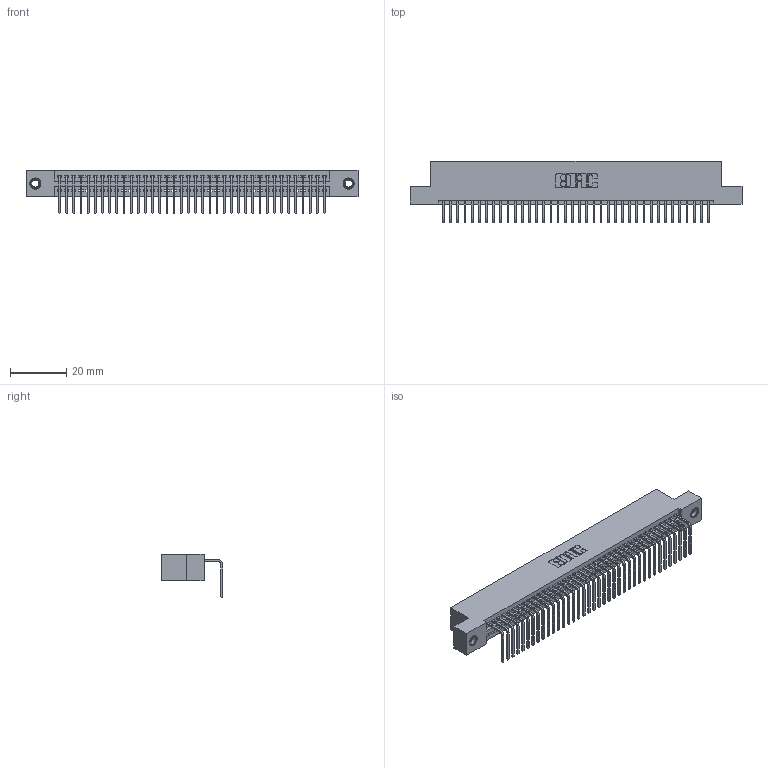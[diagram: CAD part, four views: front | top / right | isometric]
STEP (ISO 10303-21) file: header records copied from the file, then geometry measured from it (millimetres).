
FILE_DESCRIPTION (( 'STEP AP203' ), '1' );
FILE_NAME ('395-038-558-107.STEP', '2018-11-14T06:21:45', ( '' ), ( '' ), 'SwSTEP 2.0', 'SolidWorks 2016', '' );
FILE_SCHEMA (( 'CONFIG_CONTROL_DESIGN' ));
Length unit declared in the file: inch
Products named in the file (4): 345 Part_Flush Mounting Lugs - 0.156 Dia-TI; 395-038-558-107; 345-292-001_558 Tail - 2; 345-250-001_345-250-005-103
Assembly tree (41 placements, depth 2):
  395-038-558-107
    345 Part_Flush Mounting Lugs - 0.156 Dia-TI
    345-292-001_558 Tail - 2  x38
    345-250-001_345-250-005-103  x2
Bounding box: 117.73 x 21.83 x 15.37 mm (x, y, z)
Volume: 11262.3 mm3; surface area: 15688.8 mm2
Topology: 41 solids, 41 shells, 2466 faces, 7393 edges, 4870 vertices
Faces by surface type: plane 1708, cylinder 742, cone 12, torus 4
Entity records: 30408 total; most frequent: CARTESIAN_POINT 5249, ORIENTED_EDGE 5214, DIRECTION 4617, EDGE_CURVE 2607, VECTOR 2303, LINE 2303, VERTEX_POINT 1732, AXIS2_PLACEMENT_3D 1157
